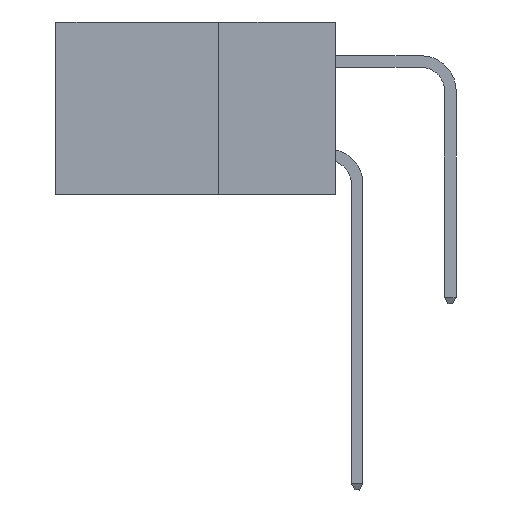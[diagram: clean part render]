
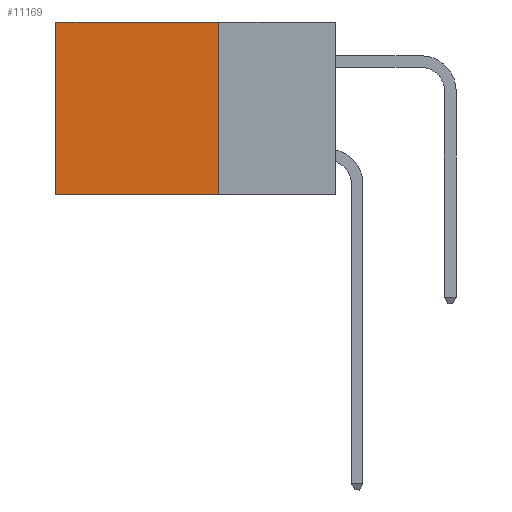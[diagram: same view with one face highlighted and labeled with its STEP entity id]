
A CAD part, left-side view. The second image highlights one B-rep face of the part: STEP entity #11169.
In plain terms, the highlighted planar face has unit normal (-1, 0, 0).
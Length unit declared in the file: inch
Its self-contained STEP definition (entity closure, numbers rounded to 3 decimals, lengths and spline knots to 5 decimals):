
#345 = CARTESIAN_POINT ( 'NONE',  ( 0.2875, 0.25, -0.37 ) ) ;
#595 = ORIENTED_EDGE ( 'NONE', *, *, #8970, .F. ) ;
#750 = VERTEX_POINT ( 'NONE', #4660 ) ;
#780 = VECTOR ( 'NONE', #3216, 39.37008 ) ;
#1853 = LINE ( 'NONE', #6297, #780 ) ;
#2486 = ORIENTED_EDGE ( 'NONE', *, *, #5799, .T. ) ;
#2498 = LINE ( 'NONE', #345, #10383 ) ;
#2552 = LINE ( 'NONE', #6946, #12468 ) ;
#3216 = DIRECTION ( 'NONE',  ( 0., 0., -1. ) ) ;
#4085 = DIRECTION ( 'NONE',  ( 0., 0., -1. ) ) ;
#4196 = CARTESIAN_POINT ( 'NONE',  ( 0.2875, 0.25, 0. ) ) ;
#4324 = CARTESIAN_POINT ( 'NONE',  ( 0.2875, 0.6, -0.37 ) ) ;
#4567 = DIRECTION ( 'NONE',  ( 0., 1., 0. ) ) ;
#4660 = CARTESIAN_POINT ( 'NONE',  ( 0.2875, 0.6, 0. ) ) ;
#4953 = FACE_OUTER_BOUND ( 'NONE', #13955, .T. ) ;
#5566 = CARTESIAN_POINT ( 'NONE',  ( 0.2875, 0.6, 0. ) ) ;
#5799 = EDGE_CURVE ( 'NONE', #11478, #750, #2552, .T. ) ;
#6297 = CARTESIAN_POINT ( 'NONE',  ( 0.2875, 0.25, 0. ) ) ;
#6946 = CARTESIAN_POINT ( 'NONE',  ( 0.2875, 0.25, 0. ) ) ;
#7016 = LINE ( 'NONE', #5566, #11906 ) ;
#7117 = PLANE ( 'NONE',  #10270 ) ;
#7441 = ORIENTED_EDGE ( 'NONE', *, *, #7610, .F. ) ;
#7610 = EDGE_CURVE ( 'NONE', #11478, #10046, #1853, .T. ) ;
#8970 = EDGE_CURVE ( 'NONE', #10046, #10062, #2498, .T. ) ;
#9352 = DIRECTION ( 'NONE',  ( 1., 0., 0. ) ) ;
#9985 = DIRECTION ( 'NONE',  ( 0., 0., -1. ) ) ;
#10046 = VERTEX_POINT ( 'NONE', #10716 ) ;
#10062 = VERTEX_POINT ( 'NONE', #4324 ) ;
#10270 = AXIS2_PLACEMENT_3D ( 'NONE', #12688, #9352, #4085 ) ;
#10383 = VECTOR ( 'NONE', #11001, 39.37008 ) ;
#10716 = CARTESIAN_POINT ( 'NONE',  ( 0.2875, 0.25, -0.37 ) ) ;
#11001 = DIRECTION ( 'NONE',  ( 0., 1., 0. ) ) ;
#11169 = ADVANCED_FACE ( 'NONE', ( #4953 ), #7117, .F. ) ;
#11478 = VERTEX_POINT ( 'NONE', #4196 ) ;
#11906 = VECTOR ( 'NONE', #9985, 39.37008 ) ;
#12468 = VECTOR ( 'NONE', #4567, 39.37008 ) ;
#12688 = CARTESIAN_POINT ( 'NONE',  ( 0.2875, 0.25, 0. ) ) ;
#13167 = EDGE_CURVE ( 'NONE', #750, #10062, #7016, .T. ) ;
#13646 = ORIENTED_EDGE ( 'NONE', *, *, #13167, .T. ) ;
#13955 = EDGE_LOOP ( 'NONE', ( #13646, #595, #7441, #2486 ) ) ;
